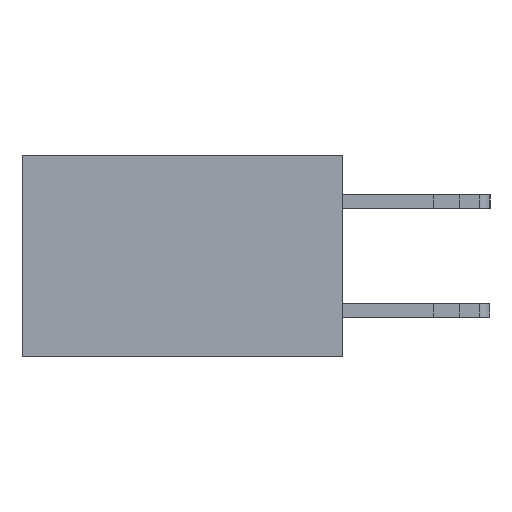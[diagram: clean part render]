
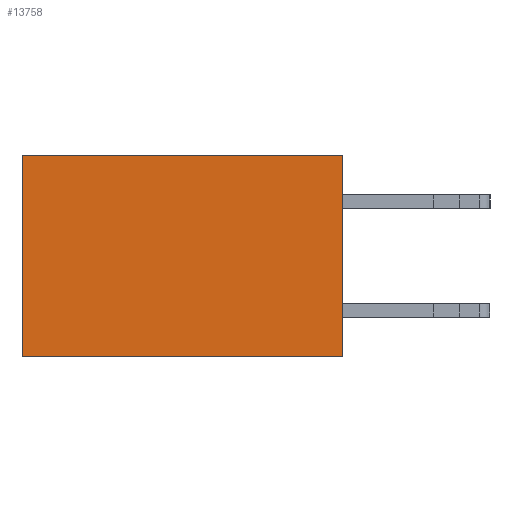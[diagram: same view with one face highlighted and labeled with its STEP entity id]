
A CAD part, left-side view. The second image highlights one B-rep face of the part: STEP entity #13758.
In plain terms, the highlighted planar face has unit normal (-1, 0, 0).
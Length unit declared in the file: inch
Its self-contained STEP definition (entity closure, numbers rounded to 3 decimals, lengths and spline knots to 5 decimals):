
#324 = DIRECTION ( 'NONE',  ( 0., 1., 0. ) ) ;
#427 = VERTEX_POINT ( 'NONE', #10179 ) ;
#826 = CARTESIAN_POINT ( 'NONE',  ( 0.277, 0., -0.37 ) ) ;
#2506 = DIRECTION ( 'NONE',  ( 1., 0., 0. ) ) ;
#2660 = ORIENTED_EDGE ( 'NONE', *, *, #17060, .T. ) ;
#2805 = ORIENTED_EDGE ( 'NONE', *, *, #16392, .F. ) ;
#3631 = VERTEX_POINT ( 'NONE', #7010 ) ;
#4027 = CARTESIAN_POINT ( 'NONE',  ( 0.277, 0.59, 0. ) ) ;
#4895 = VECTOR ( 'NONE', #7561, 39.37008 ) ;
#5579 = LINE ( 'NONE', #18094, #18376 ) ;
#5852 = CARTESIAN_POINT ( 'NONE',  ( 0.277, 0., -0.37 ) ) ;
#6462 = LINE ( 'NONE', #14546, #7012 ) ;
#6484 = AXIS2_PLACEMENT_3D ( 'NONE', #826, #2506, #13987 ) ;
#7010 = CARTESIAN_POINT ( 'NONE',  ( 0.277, 0., -0.37 ) ) ;
#7012 = VECTOR ( 'NONE', #14672, 39.37008 ) ;
#7234 = VERTEX_POINT ( 'NONE', #19772 ) ;
#7561 = DIRECTION ( 'NONE',  ( 0., 0., -1. ) ) ;
#8091 = ORIENTED_EDGE ( 'NONE', *, *, #8570, .T. ) ;
#8570 = EDGE_CURVE ( 'NONE', #12275, #7234, #6462, .T. ) ;
#9296 = VECTOR ( 'NONE', #17343, 39.37008 ) ;
#9793 = LINE ( 'NONE', #12571, #9296 ) ;
#10179 = CARTESIAN_POINT ( 'NONE',  ( 0.277, 0., 0. ) ) ;
#11474 = FACE_OUTER_BOUND ( 'NONE', #15724, .T. ) ;
#12101 = LINE ( 'NONE', #5852, #4895 ) ;
#12116 = EDGE_CURVE ( 'NONE', #3631, #7234, #5579, .T. ) ;
#12275 = VERTEX_POINT ( 'NONE', #4027 ) ;
#12382 = PLANE ( 'NONE',  #6484 ) ;
#12571 = CARTESIAN_POINT ( 'NONE',  ( 0.277, 0., 0. ) ) ;
#13108 = ORIENTED_EDGE ( 'NONE', *, *, #12116, .F. ) ;
#13758 = ADVANCED_FACE ( 'NONE', ( #11474 ), #12382, .F. ) ;
#13987 = DIRECTION ( 'NONE',  ( 0., 0., -1. ) ) ;
#14546 = CARTESIAN_POINT ( 'NONE',  ( 0.277, 0.59, -0.37 ) ) ;
#14672 = DIRECTION ( 'NONE',  ( 0., 0., -1. ) ) ;
#15724 = EDGE_LOOP ( 'NONE', ( #8091, #13108, #2805, #2660 ) ) ;
#16392 = EDGE_CURVE ( 'NONE', #427, #3631, #12101, .T. ) ;
#17060 = EDGE_CURVE ( 'NONE', #427, #12275, #9793, .T. ) ;
#17343 = DIRECTION ( 'NONE',  ( 0., 1., 0. ) ) ;
#18094 = CARTESIAN_POINT ( 'NONE',  ( 0.277, 0., -0.37 ) ) ;
#18376 = VECTOR ( 'NONE', #324, 39.37008 ) ;
#19772 = CARTESIAN_POINT ( 'NONE',  ( 0.277, 0.59, -0.37 ) ) ;
